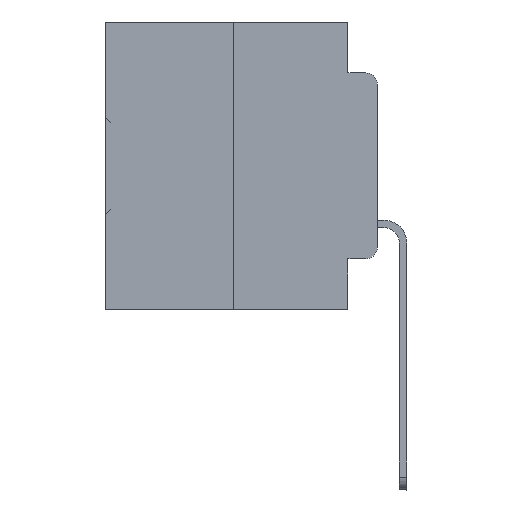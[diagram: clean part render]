
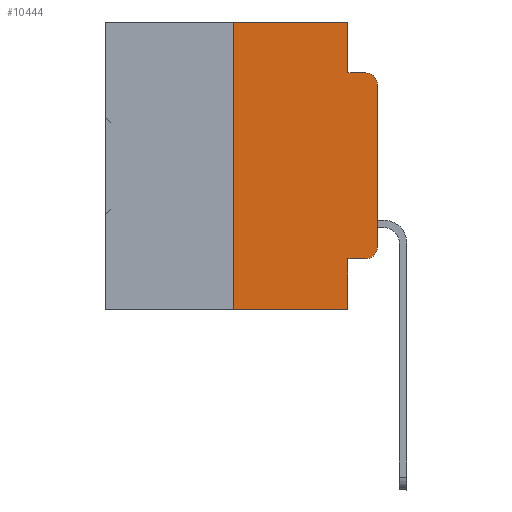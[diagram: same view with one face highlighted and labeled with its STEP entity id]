
A CAD part, left-side view. The second image highlights one B-rep face of the part: STEP entity #10444.
In plain terms, the highlighted planar face has unit normal (-1, 0, 0).
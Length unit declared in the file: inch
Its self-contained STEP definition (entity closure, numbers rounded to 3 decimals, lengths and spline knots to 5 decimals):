
#756 = CARTESIAN_POINT ( 'NONE',  ( 0., 0.473, -0.5 ) ) ;
#821 = DIRECTION ( 'NONE',  ( 0., 0., -1. ) ) ;
#1357 = ORIENTED_EDGE ( 'NONE', *, *, #31756, .T. ) ;
#1360 = VERTEX_POINT ( 'NONE', #12897 ) ;
#1828 = EDGE_CURVE ( 'NONE', #26594, #33270, #35842, .T. ) ;
#2639 = VERTEX_POINT ( 'NONE', #32302 ) ;
#2687 = VERTEX_POINT ( 'NONE', #26955 ) ;
#3222 = DIRECTION ( 'NONE',  ( 0., 0., -1. ) ) ;
#3281 = LINE ( 'NONE', #8763, #7199 ) ;
#3866 = VERTEX_POINT ( 'NONE', #32450 ) ;
#4367 = VERTEX_POINT ( 'NONE', #35045 ) ;
#4753 = DIRECTION ( 'NONE',  ( 0., 0., -1. ) ) ;
#5243 = CARTESIAN_POINT ( 'NONE',  ( 0., 0.051, 0. ) ) ;
#5304 = VECTOR ( 'NONE', #14099, 39.37008 ) ;
#5565 = AXIS2_PLACEMENT_3D ( 'NONE', #25351, #8620, #22081 ) ;
#5892 = CARTESIAN_POINT ( 'NONE',  ( 0., 0.02, -0.3915 ) ) ;
#7199 = VECTOR ( 'NONE', #33857, 39.37008 ) ;
#7425 = CARTESIAN_POINT ( 'NONE',  ( 0., 0.473, 0. ) ) ;
#7671 = ORIENTED_EDGE ( 'NONE', *, *, #25712, .T. ) ;
#7870 = LINE ( 'NONE', #5243, #17079 ) ;
#8620 = DIRECTION ( 'NONE',  ( -1., 0., 0. ) ) ;
#8763 = CARTESIAN_POINT ( 'NONE',  ( 0., 0.051, -0.0885 ) ) ;
#9084 = VERTEX_POINT ( 'NONE', #13575 ) ;
#10444 = ADVANCED_FACE ( 'NONE', ( #29538 ), #25594, .F. ) ;
#10525 = DIRECTION ( 'NONE',  ( 0., -1., 0. ) ) ;
#10560 = LINE ( 'NONE', #19970, #5304 ) ;
#10940 = AXIS2_PLACEMENT_3D ( 'NONE', #5892, #24823, #30274 ) ;
#10965 = LINE ( 'NONE', #756, #13981 ) ;
#12012 = CARTESIAN_POINT ( 'NONE',  ( 0., 0.051, -0.0885 ) ) ;
#12897 = CARTESIAN_POINT ( 'NONE',  ( 0., 0., -0.3915 ) ) ;
#13575 = CARTESIAN_POINT ( 'NONE',  ( 0., 0.051, -0.5 ) ) ;
#13981 = VECTOR ( 'NONE', #14446, 39.37008 ) ;
#14061 = VECTOR ( 'NONE', #32614, 39.37008 ) ;
#14099 = DIRECTION ( 'NONE',  ( 0., -1., 0. ) ) ;
#14446 = DIRECTION ( 'NONE',  ( 0., -1., 0. ) ) ;
#14479 = CARTESIAN_POINT ( 'NONE',  ( 0., 0.25, -0.5 ) ) ;
#14919 = ORIENTED_EDGE ( 'NONE', *, *, #31383, .F. ) ;
#15638 = DIRECTION ( 'NONE',  ( 0., 0., 1. ) ) ;
#16629 = VECTOR ( 'NONE', #10525, 39.37008 ) ;
#16959 = LINE ( 'NONE', #28624, #23500 ) ;
#17079 = VECTOR ( 'NONE', #4753, 39.37008 ) ;
#17173 = DIRECTION ( 'NONE',  ( 1., 0., 0. ) ) ;
#17779 = CIRCLE ( 'NONE', #5565, 0.02 ) ;
#17851 = CIRCLE ( 'NONE', #10940, 0.02 ) ;
#17993 = ORIENTED_EDGE ( 'NONE', *, *, #1828, .F. ) ;
#18149 = CARTESIAN_POINT ( 'NONE',  ( 0., 0.051, 0. ) ) ;
#18706 = CARTESIAN_POINT ( 'NONE',  ( 0., 0.25, 0. ) ) ;
#18824 = EDGE_CURVE ( 'NONE', #34423, #3866, #3281, .T. ) ;
#19791 = ORIENTED_EDGE ( 'NONE', *, *, #29264, .T. ) ;
#19970 = CARTESIAN_POINT ( 'NONE',  ( 0., 0.051, -0.4115 ) ) ;
#20220 = ORIENTED_EDGE ( 'NONE', *, *, #18824, .F. ) ;
#21032 = EDGE_LOOP ( 'NONE', ( #30621, #1357, #20220, #14919, #33090, #17993, #7671, #25937, #19791, #35299 ) ) ;
#21268 = EDGE_CURVE ( 'NONE', #1360, #2687, #35825, .T. ) ;
#21298 = CARTESIAN_POINT ( 'NONE',  ( 0., 0., 0. ) ) ;
#22081 = DIRECTION ( 'NONE',  ( 0., 0., -1. ) ) ;
#22139 = EDGE_CURVE ( 'NONE', #4367, #9084, #7870, .T. ) ;
#23500 = VECTOR ( 'NONE', #821, 39.37008 ) ;
#24823 = DIRECTION ( 'NONE',  ( -1., 0., 0. ) ) ;
#24841 = AXIS2_PLACEMENT_3D ( 'NONE', #33938, #17173, #3222 ) ;
#25351 = CARTESIAN_POINT ( 'NONE',  ( 0., 0.02, -0.1085 ) ) ;
#25410 = VERTEX_POINT ( 'NONE', #18149 ) ;
#25594 = PLANE ( 'NONE',  #24841 ) ;
#25712 = EDGE_CURVE ( 'NONE', #26594, #9084, #10965, .T. ) ;
#25937 = ORIENTED_EDGE ( 'NONE', *, *, #22139, .F. ) ;
#26594 = VERTEX_POINT ( 'NONE', #14479 ) ;
#26955 = CARTESIAN_POINT ( 'NONE',  ( 0., 0., -0.1085 ) ) ;
#28624 = CARTESIAN_POINT ( 'NONE',  ( 0., 0.051, 0. ) ) ;
#29264 = EDGE_CURVE ( 'NONE', #4367, #2639, #10560, .T. ) ;
#29538 = FACE_OUTER_BOUND ( 'NONE', #21032, .T. ) ;
#30274 = DIRECTION ( 'NONE',  ( 0., 0., -1. ) ) ;
#30621 = ORIENTED_EDGE ( 'NONE', *, *, #21268, .T. ) ;
#30645 = EDGE_CURVE ( 'NONE', #2639, #1360, #17851, .T. ) ;
#31383 = EDGE_CURVE ( 'NONE', #25410, #34423, #16959, .T. ) ;
#31756 = EDGE_CURVE ( 'NONE', #2687, #3866, #17779, .T. ) ;
#32276 = LINE ( 'NONE', #7425, #16629 ) ;
#32302 = CARTESIAN_POINT ( 'NONE',  ( 0., 0.02, -0.4115 ) ) ;
#32450 = CARTESIAN_POINT ( 'NONE',  ( 0., 0.02, -0.0885 ) ) ;
#32614 = DIRECTION ( 'NONE',  ( 0., 0., 1. ) ) ;
#32994 = CARTESIAN_POINT ( 'NONE',  ( 0., 0.25, 0. ) ) ;
#33090 = ORIENTED_EDGE ( 'NONE', *, *, #35362, .F. ) ;
#33270 = VERTEX_POINT ( 'NONE', #18706 ) ;
#33687 = VECTOR ( 'NONE', #15638, 39.37008 ) ;
#33857 = DIRECTION ( 'NONE',  ( 0., -1., 0. ) ) ;
#33938 = CARTESIAN_POINT ( 'NONE',  ( 0., 0.473, 0. ) ) ;
#34423 = VERTEX_POINT ( 'NONE', #12012 ) ;
#35045 = CARTESIAN_POINT ( 'NONE',  ( 0., 0.051, -0.4115 ) ) ;
#35299 = ORIENTED_EDGE ( 'NONE', *, *, #30645, .T. ) ;
#35362 = EDGE_CURVE ( 'NONE', #33270, #25410, #32276, .T. ) ;
#35825 = LINE ( 'NONE', #21298, #33687 ) ;
#35842 = LINE ( 'NONE', #32994, #14061 ) ;
